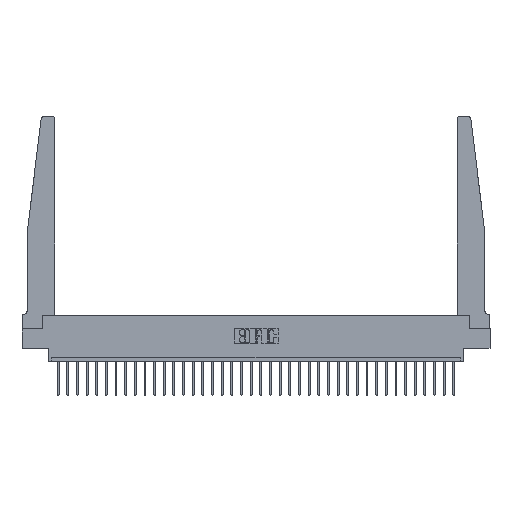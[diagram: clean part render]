
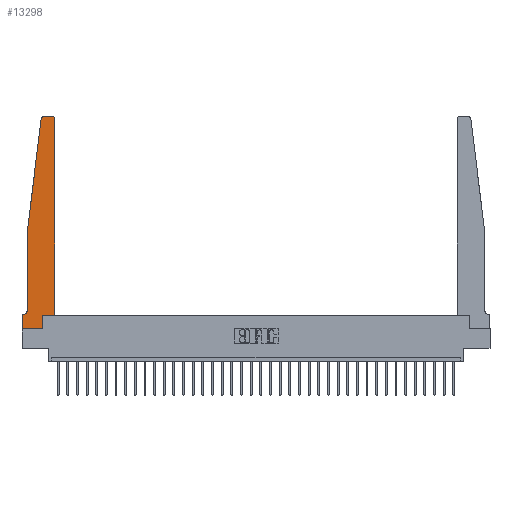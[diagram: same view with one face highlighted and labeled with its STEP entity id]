
A CAD part, top view. The second image highlights one B-rep face of the part: STEP entity #13298.
In plain terms, the highlighted planar face has unit normal (0, 0, 1).
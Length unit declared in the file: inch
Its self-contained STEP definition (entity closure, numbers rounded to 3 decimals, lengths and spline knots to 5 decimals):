
#13 = CARTESIAN_POINT ( 'NONE',  ( 0.2605, 0.18, 0.37 ) ) ;
#28 = LINE ( 'NONE', #21649, #20998 ) ;
#269 = DIRECTION ( 'NONE',  ( 0., 1., 0. ) ) ;
#608 = ORIENTED_EDGE ( 'NONE', *, *, #4094, .T. ) ;
#809 = CIRCLE ( 'NONE', #19632, 0.03 ) ;
#878 = EDGE_CURVE ( 'NONE', #27682, #5917, #19390, .T. ) ;
#1135 = ORIENTED_EDGE ( 'NONE', *, *, #5189, .T. ) ;
#1338 = DIRECTION ( 'NONE',  ( 1., 0., 0. ) ) ;
#1800 = VERTEX_POINT ( 'NONE', #12825 ) ;
#1870 = VECTOR ( 'NONE', #269, 39.37008 ) ;
#2584 = DIRECTION ( 'NONE',  ( -0.122, -0.992, 0. ) ) ;
#2921 = VERTEX_POINT ( 'NONE', #18912 ) ;
#3158 = VERTEX_POINT ( 'NONE', #8691 ) ;
#3439 = CARTESIAN_POINT ( 'NONE',  ( 0.25, 2.75, 0.37 ) ) ;
#3696 = EDGE_CURVE ( 'NONE', #5917, #22540, #15691, .T. ) ;
#3882 = VERTEX_POINT ( 'NONE', #28554 ) ;
#4094 = EDGE_CURVE ( 'NONE', #17191, #12350, #28050, .T. ) ;
#4155 = ORIENTED_EDGE ( 'NONE', *, *, #878, .T. ) ;
#4457 = EDGE_CURVE ( 'NONE', #2921, #17191, #17370, .T. ) ;
#5189 = EDGE_CURVE ( 'NONE', #30285, #1800, #25573, .T. ) ;
#5591 = ORIENTED_EDGE ( 'NONE', *, *, #21457, .T. ) ;
#5917 = VERTEX_POINT ( 'NONE', #10625 ) ;
#6189 = DIRECTION ( 'NONE',  ( 0., 0., 1. ) ) ;
#6669 = PLANE ( 'NONE',  #8497 ) ;
#6687 = EDGE_LOOP ( 'NONE', ( #29536, #8289, #31379, #13590, #1135, #10903, #5591, #13600, #8427, #608, #9274, #4155 ) ) ;
#8289 = ORIENTED_EDGE ( 'NONE', *, *, #17491, .T. ) ;
#8427 = ORIENTED_EDGE ( 'NONE', *, *, #4457, .T. ) ;
#8497 = AXIS2_PLACEMENT_3D ( 'NONE', #11617, #6189, #26219 ) ;
#8691 = CARTESIAN_POINT ( 'NONE',  ( 0.24675, 2.72367, 0.37 ) ) ;
#8901 = CARTESIAN_POINT ( 'NONE',  ( 0.065, 0.1875, 0.37 ) ) ;
#9274 = ORIENTED_EDGE ( 'NONE', *, *, #18484, .T. ) ;
#9603 = CARTESIAN_POINT ( 'NONE',  ( 0., 0., 0.37 ) ) ;
#10047 = CARTESIAN_POINT ( 'NONE',  ( 0.065, 1.25, 0.37 ) ) ;
#10625 = CARTESIAN_POINT ( 'NONE',  ( 0.395, 2.75, 0.37 ) ) ;
#10899 = CARTESIAN_POINT ( 'NONE',  ( 0.425, 0.18, 0.37 ) ) ;
#10903 = ORIENTED_EDGE ( 'NONE', *, *, #14564, .T. ) ;
#11027 = DIRECTION ( 'NONE',  ( -1., 0., 0. ) ) ;
#11617 = CARTESIAN_POINT ( 'NONE',  ( 0., 0.1875, 0.37 ) ) ;
#12057 = LINE ( 'NONE', #17146, #1870 ) ;
#12060 = VERTEX_POINT ( 'NONE', #25399 ) ;
#12350 = VERTEX_POINT ( 'NONE', #23127 ) ;
#12753 = VERTEX_POINT ( 'NONE', #23703 ) ;
#12825 = CARTESIAN_POINT ( 'NONE',  ( 0.015, 0.1875, 0.37 ) ) ;
#12842 = VECTOR ( 'NONE', #30445, 39.37008 ) ;
#13159 = EDGE_CURVE ( 'NONE', #12060, #30285, #30980, .T. ) ;
#13298 = ADVANCED_FACE ( 'NONE', ( #23529 ), #6669, .T. ) ;
#13590 = ORIENTED_EDGE ( 'NONE', *, *, #13159, .T. ) ;
#13600 = ORIENTED_EDGE ( 'NONE', *, *, #25808, .T. ) ;
#14225 = LINE ( 'NONE', #9603, #24908 ) ;
#14290 = CARTESIAN_POINT ( 'NONE',  ( 0.425, 2.72, 0.37 ) ) ;
#14564 = EDGE_CURVE ( 'NONE', #1800, #12753, #21130, .T. ) ;
#15066 = CARTESIAN_POINT ( 'NONE',  ( 0.27653, 2.75, 0.37 ) ) ;
#15114 = EDGE_CURVE ( 'NONE', #3158, #12060, #21810, .T. ) ;
#15691 = LINE ( 'NONE', #3439, #12842 ) ;
#16271 = DIRECTION ( 'NONE',  ( 0., 0., 1. ) ) ;
#16348 = AXIS2_PLACEMENT_3D ( 'NONE', #23352, #25901, #27651 ) ;
#16447 = DIRECTION ( 'NONE',  ( 0., -1., 0. ) ) ;
#17146 = CARTESIAN_POINT ( 'NONE',  ( 0.425, 0.18, 0.37 ) ) ;
#17191 = VERTEX_POINT ( 'NONE', #30390 ) ;
#17370 = LINE ( 'NONE', #13, #29608 ) ;
#17491 = EDGE_CURVE ( 'NONE', #22540, #3158, #809, .T. ) ;
#18484 = EDGE_CURVE ( 'NONE', #12350, #27682, #12057, .T. ) ;
#18814 = DIRECTION ( 'NONE',  ( 1., 0., 0. ) ) ;
#18912 = CARTESIAN_POINT ( 'NONE',  ( 0.2605, 0., 0.37 ) ) ;
#18937 = VECTOR ( 'NONE', #1338, 39.37008 ) ;
#18982 = AXIS2_PLACEMENT_3D ( 'NONE', #19637, #29304, #11027 ) ;
#19268 = DIRECTION ( 'NONE',  ( 0., 1., 0. ) ) ;
#19390 = CIRCLE ( 'NONE', #16348, 0.03 ) ;
#19575 = CARTESIAN_POINT ( 'NONE',  ( 0.065, 0.2375, 0.37 ) ) ;
#19632 = AXIS2_PLACEMENT_3D ( 'NONE', #20885, #16271, #18814 ) ;
#19637 = CARTESIAN_POINT ( 'NONE',  ( 0.015, 0.2375, 0.37 ) ) ;
#20046 = DIRECTION ( 'NONE',  ( 0., -1., 0. ) ) ;
#20282 = VECTOR ( 'NONE', #2584, 39.37008 ) ;
#20885 = CARTESIAN_POINT ( 'NONE',  ( 0.27653, 2.72, 0.37 ) ) ;
#20998 = VECTOR ( 'NONE', #27078, 39.37008 ) ;
#21130 = LINE ( 'NONE', #8901, #23301 ) ;
#21457 = EDGE_CURVE ( 'NONE', #12753, #3882, #14225, .T. ) ;
#21649 = CARTESIAN_POINT ( 'NONE',  ( 0., 0., 0.37 ) ) ;
#21810 = LINE ( 'NONE', #10047, #20282 ) ;
#22540 = VERTEX_POINT ( 'NONE', #15066 ) ;
#23127 = CARTESIAN_POINT ( 'NONE',  ( 0.425, 0.18, 0.37 ) ) ;
#23301 = VECTOR ( 'NONE', #30817, 39.37008 ) ;
#23352 = CARTESIAN_POINT ( 'NONE',  ( 0.395, 2.72, 0.37 ) ) ;
#23529 = FACE_OUTER_BOUND ( 'NONE', #6687, .T. ) ;
#23703 = CARTESIAN_POINT ( 'NONE',  ( 0., 0.1875, 0.37 ) ) ;
#24908 = VECTOR ( 'NONE', #16447, 39.37008 ) ;
#25399 = CARTESIAN_POINT ( 'NONE',  ( 0.065, 1.25, 0.37 ) ) ;
#25573 = CIRCLE ( 'NONE', #18982, 0.05 ) ;
#25808 = EDGE_CURVE ( 'NONE', #3882, #2921, #28, .T. ) ;
#25901 = DIRECTION ( 'NONE',  ( 0., 0., 1. ) ) ;
#26219 = DIRECTION ( 'NONE',  ( 1., 0., 0. ) ) ;
#27078 = DIRECTION ( 'NONE',  ( 1., 0., 0. ) ) ;
#27651 = DIRECTION ( 'NONE',  ( 1., 0., 0. ) ) ;
#27682 = VERTEX_POINT ( 'NONE', #14290 ) ;
#28050 = LINE ( 'NONE', #10899, #18937 ) ;
#28554 = CARTESIAN_POINT ( 'NONE',  ( 0., 0., 0.37 ) ) ;
#29304 = DIRECTION ( 'NONE',  ( 0., 0., -1. ) ) ;
#29536 = ORIENTED_EDGE ( 'NONE', *, *, #3696, .T. ) ;
#29608 = VECTOR ( 'NONE', #19268, 39.37008 ) ;
#29738 = CARTESIAN_POINT ( 'NONE',  ( 0.065, 1.25, 0.37 ) ) ;
#29820 = VECTOR ( 'NONE', #20046, 39.37008 ) ;
#30285 = VERTEX_POINT ( 'NONE', #19575 ) ;
#30390 = CARTESIAN_POINT ( 'NONE',  ( 0.2605, 0.18, 0.37 ) ) ;
#30445 = DIRECTION ( 'NONE',  ( -1., 0., 0. ) ) ;
#30817 = DIRECTION ( 'NONE',  ( -1., 0., 0. ) ) ;
#30980 = LINE ( 'NONE', #29738, #29820 ) ;
#31379 = ORIENTED_EDGE ( 'NONE', *, *, #15114, .T. ) ;
